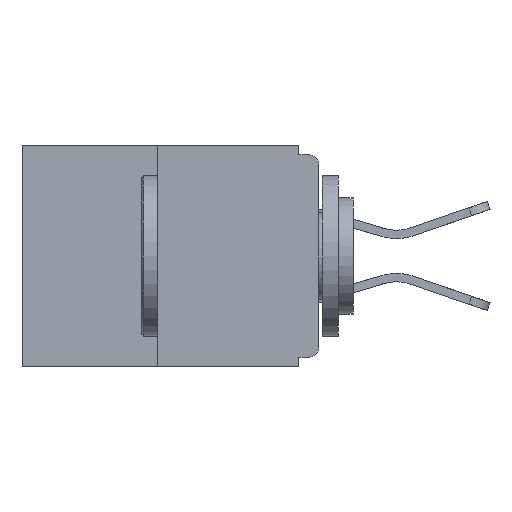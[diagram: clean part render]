
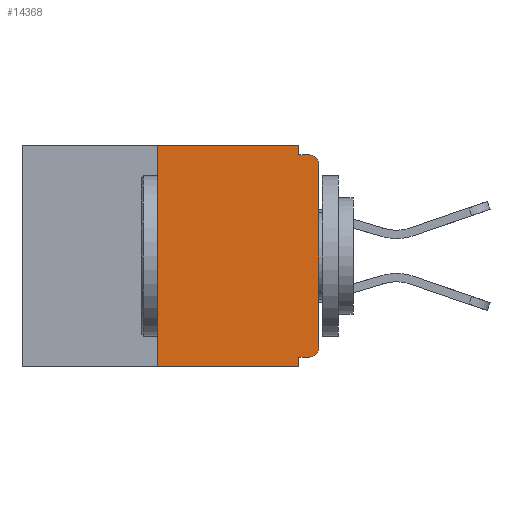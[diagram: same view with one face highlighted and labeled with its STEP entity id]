
A CAD part, left-side view. The second image highlights one B-rep face of the part: STEP entity #14368.
In plain terms, the highlighted planar face has unit normal (-1, 0, 0).
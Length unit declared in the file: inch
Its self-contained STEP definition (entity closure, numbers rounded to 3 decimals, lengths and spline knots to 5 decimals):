
#126 = PLANE ( 'NONE',  #10389 ) ;
#199 = ORIENTED_EDGE ( 'NONE', *, *, #13537, .F. ) ;
#206 = CIRCLE ( 'NONE', #13778, 0.015 ) ;
#391 = ORIENTED_EDGE ( 'NONE', *, *, #1967, .T. ) ;
#794 = VERTEX_POINT ( 'NONE', #12431 ) ;
#897 = VERTEX_POINT ( 'NONE', #21084 ) ;
#1174 = LINE ( 'NONE', #14973, #18101 ) ;
#1287 = CIRCLE ( 'NONE', #6200, 0.015 ) ;
#1588 = CARTESIAN_POINT ( 'NONE',  ( 0., 0.015, -0.03 ) ) ;
#1801 = ORIENTED_EDGE ( 'NONE', *, *, #4914, .F. ) ;
#1967 = EDGE_CURVE ( 'NONE', #5255, #16556, #206, .T. ) ;
#2017 = CARTESIAN_POINT ( 'NONE',  ( 0., 0.46, 0. ) ) ;
#2051 = ORIENTED_EDGE ( 'NONE', *, *, #17723, .T. ) ;
#2491 = ORIENTED_EDGE ( 'NONE', *, *, #8633, .F. ) ;
#2838 = CARTESIAN_POINT ( 'NONE',  ( 0., 0.25, 0. ) ) ;
#2862 = LINE ( 'NONE', #14659, #16446 ) ;
#3301 = DIRECTION ( 'NONE',  ( 0., -1., 0. ) ) ;
#3377 = CARTESIAN_POINT ( 'NONE',  ( 0., 0.46, -0.343 ) ) ;
#3774 = FACE_OUTER_BOUND ( 'NONE', #18550, .T. ) ;
#3911 = EDGE_CURVE ( 'NONE', #14704, #8772, #11414, .T. ) ;
#4228 = CARTESIAN_POINT ( 'NONE',  ( 0., 0.46, 0. ) ) ;
#4468 = DIRECTION ( 'NONE',  ( -1., 0., 0. ) ) ;
#4876 = DIRECTION ( 'NONE',  ( 0., 0., -1. ) ) ;
#4907 = DIRECTION ( 'NONE',  ( -1., 0., 0. ) ) ;
#4914 = EDGE_CURVE ( 'NONE', #11201, #14704, #1174, .T. ) ;
#5059 = CARTESIAN_POINT ( 'NONE',  ( 0., 0., -0.03 ) ) ;
#5255 = VERTEX_POINT ( 'NONE', #5059 ) ;
#6097 = DIRECTION ( 'NONE',  ( 0., 0., -1. ) ) ;
#6200 = AXIS2_PLACEMENT_3D ( 'NONE', #15827, #4468, #6097 ) ;
#6345 = VERTEX_POINT ( 'NONE', #18234 ) ;
#6506 = CARTESIAN_POINT ( 'NONE',  ( 0., 0.015, -0.328 ) ) ;
#6681 = DIRECTION ( 'NONE',  ( 1., 0., 0. ) ) ;
#6893 = LINE ( 'NONE', #20715, #15092 ) ;
#6966 = DIRECTION ( 'NONE',  ( 0., 0., -1. ) ) ;
#7164 = LINE ( 'NONE', #8116, #13269 ) ;
#7260 = DIRECTION ( 'NONE',  ( 0., -1., 0. ) ) ;
#8114 = VECTOR ( 'NONE', #9077, 39.37008 ) ;
#8116 = CARTESIAN_POINT ( 'NONE',  ( 0., 0.25, 0. ) ) ;
#8314 = CARTESIAN_POINT ( 'NONE',  ( 0., 0.031, -0.328 ) ) ;
#8633 = EDGE_CURVE ( 'NONE', #11538, #12076, #11664, .T. ) ;
#8772 = VERTEX_POINT ( 'NONE', #19600 ) ;
#9077 = DIRECTION ( 'NONE',  ( 0., -1., 0. ) ) ;
#9320 = DIRECTION ( 'NONE',  ( 0., 0., 1. ) ) ;
#9659 = DIRECTION ( 'NONE',  ( 0., 0., 1. ) ) ;
#10389 = AXIS2_PLACEMENT_3D ( 'NONE', #2017, #6681, #6966 ) ;
#11182 = EDGE_CURVE ( 'NONE', #12076, #794, #2862, .T. ) ;
#11201 = VERTEX_POINT ( 'NONE', #6506 ) ;
#11414 = LINE ( 'NONE', #16657, #16047 ) ;
#11441 = ORIENTED_EDGE ( 'NONE', *, *, #3911, .F. ) ;
#11538 = VERTEX_POINT ( 'NONE', #2838 ) ;
#11664 = LINE ( 'NONE', #4228, #8114 ) ;
#11751 = DIRECTION ( 'NONE',  ( 0., 0., -1. ) ) ;
#11921 = CARTESIAN_POINT ( 'NONE',  ( 0., 0.031, 0. ) ) ;
#12076 = VERTEX_POINT ( 'NONE', #11921 ) ;
#12431 = CARTESIAN_POINT ( 'NONE',  ( 0., 0.031, -0.015 ) ) ;
#12642 = EDGE_CURVE ( 'NONE', #794, #16556, #12764, .T. ) ;
#12764 = LINE ( 'NONE', #17056, #19959 ) ;
#12883 = DIRECTION ( 'NONE',  ( 0., 0., -1. ) ) ;
#13269 = VECTOR ( 'NONE', #9659, 39.37008 ) ;
#13537 = EDGE_CURVE ( 'NONE', #6345, #11538, #7164, .T. ) ;
#13778 = AXIS2_PLACEMENT_3D ( 'NONE', #1588, #4907, #12883 ) ;
#14368 = ADVANCED_FACE ( 'NONE', ( #3774 ), #126, .F. ) ;
#14412 = ORIENTED_EDGE ( 'NONE', *, *, #12642, .F. ) ;
#14659 = CARTESIAN_POINT ( 'NONE',  ( 0., 0.031, 0. ) ) ;
#14704 = VERTEX_POINT ( 'NONE', #8314 ) ;
#14973 = CARTESIAN_POINT ( 'NONE',  ( 0., 0., -0.328 ) ) ;
#15092 = VECTOR ( 'NONE', #9320, 39.37008 ) ;
#15484 = ORIENTED_EDGE ( 'NONE', *, *, #11182, .F. ) ;
#15827 = CARTESIAN_POINT ( 'NONE',  ( 0., 0.015, -0.313 ) ) ;
#16047 = VECTOR ( 'NONE', #11751, 39.37008 ) ;
#16446 = VECTOR ( 'NONE', #4876, 39.37008 ) ;
#16556 = VERTEX_POINT ( 'NONE', #19203 ) ;
#16657 = CARTESIAN_POINT ( 'NONE',  ( 0., 0.031, -0.343 ) ) ;
#17056 = CARTESIAN_POINT ( 'NONE',  ( 0., 0., -0.015 ) ) ;
#17723 = EDGE_CURVE ( 'NONE', #11201, #897, #1287, .T. ) ;
#17997 = ORIENTED_EDGE ( 'NONE', *, *, #19633, .T. ) ;
#18101 = VECTOR ( 'NONE', #18121, 39.37008 ) ;
#18121 = DIRECTION ( 'NONE',  ( 0., 1., 0. ) ) ;
#18234 = CARTESIAN_POINT ( 'NONE',  ( 0., 0.25, -0.343 ) ) ;
#18241 = VECTOR ( 'NONE', #3301, 39.37008 ) ;
#18529 = LINE ( 'NONE', #3377, #18241 ) ;
#18550 = EDGE_LOOP ( 'NONE', ( #2491, #199, #20700, #11441, #1801, #2051, #17997, #391, #14412, #15484 ) ) ;
#19203 = CARTESIAN_POINT ( 'NONE',  ( 0., 0.015, -0.015 ) ) ;
#19600 = CARTESIAN_POINT ( 'NONE',  ( 0., 0.031, -0.343 ) ) ;
#19633 = EDGE_CURVE ( 'NONE', #897, #5255, #6893, .T. ) ;
#19959 = VECTOR ( 'NONE', #7260, 39.37008 ) ;
#20417 = EDGE_CURVE ( 'NONE', #6345, #8772, #18529, .T. ) ;
#20700 = ORIENTED_EDGE ( 'NONE', *, *, #20417, .T. ) ;
#20715 = CARTESIAN_POINT ( 'NONE',  ( 0., 0., 0. ) ) ;
#21084 = CARTESIAN_POINT ( 'NONE',  ( 0., 0., -0.313 ) ) ;
